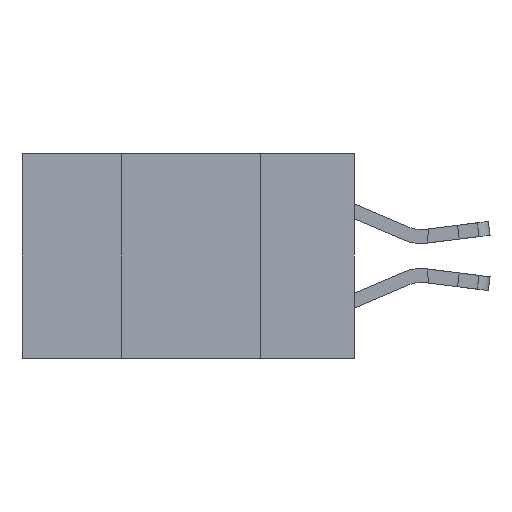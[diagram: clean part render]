
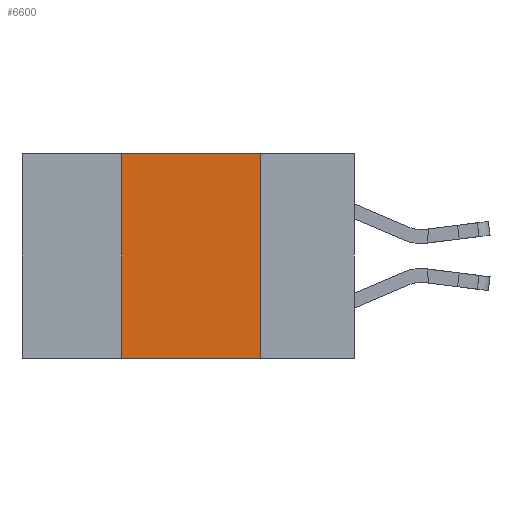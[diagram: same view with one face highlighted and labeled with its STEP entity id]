
A CAD part, left-side view. The second image highlights one B-rep face of the part: STEP entity #6600.
In plain terms, the highlighted planar face has unit normal (-1, 0, 0).
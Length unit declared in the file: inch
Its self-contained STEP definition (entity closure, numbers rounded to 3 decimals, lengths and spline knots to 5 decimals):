
#204 = CARTESIAN_POINT ( 'NONE',  ( 0., 0.6, 0. ) ) ;
#1066 = PLANE ( 'NONE',  #12484 ) ;
#1134 = CARTESIAN_POINT ( 'NONE',  ( 0., 0.42, -0.37 ) ) ;
#1773 = ORIENTED_EDGE ( 'NONE', *, *, #10359, .F. ) ;
#2123 = CARTESIAN_POINT ( 'NONE',  ( 0., 0.6, 0. ) ) ;
#2217 = VERTEX_POINT ( 'NONE', #1134 ) ;
#2220 = LINE ( 'NONE', #12725, #7137 ) ;
#2248 = EDGE_CURVE ( 'NONE', #2217, #8359, #2408, .T. ) ;
#2329 = EDGE_CURVE ( 'NONE', #2217, #6761, #12597, .T. ) ;
#2330 = DIRECTION ( 'NONE',  ( 0., -1., 0. ) ) ;
#2408 = LINE ( 'NONE', #5326, #4880 ) ;
#2549 = FACE_OUTER_BOUND ( 'NONE', #2796, .T. ) ;
#2796 = EDGE_LOOP ( 'NONE', ( #1773, #10125, #4559, #6039 ) ) ;
#3170 = DIRECTION ( 'NONE',  ( 0., 0., -1. ) ) ;
#4559 = ORIENTED_EDGE ( 'NONE', *, *, #2329, .F. ) ;
#4647 = LINE ( 'NONE', #204, #12364 ) ;
#4880 = VECTOR ( 'NONE', #7467, 39.37008 ) ;
#5326 = CARTESIAN_POINT ( 'NONE',  ( 0., 0.6, -0.37 ) ) ;
#5507 = CARTESIAN_POINT ( 'NONE',  ( 0., 0.42, -0.37 ) ) ;
#6039 = ORIENTED_EDGE ( 'NONE', *, *, #2248, .T. ) ;
#6412 = DIRECTION ( 'NONE',  ( 0., 0., -1. ) ) ;
#6554 = DIRECTION ( 'NONE',  ( 0., 0., 1. ) ) ;
#6600 = ADVANCED_FACE ( 'NONE', ( #2549 ), #1066, .F. ) ;
#6761 = VERTEX_POINT ( 'NONE', #11802 ) ;
#7137 = VECTOR ( 'NONE', #6412, 39.37008 ) ;
#7467 = DIRECTION ( 'NONE',  ( 0., -1., 0. ) ) ;
#8359 = VERTEX_POINT ( 'NONE', #10468 ) ;
#9397 = CARTESIAN_POINT ( 'NONE',  ( 0., 0.17, 0. ) ) ;
#9456 = DIRECTION ( 'NONE',  ( 1., 0., 0. ) ) ;
#9756 = EDGE_CURVE ( 'NONE', #6761, #10270, #4647, .T. ) ;
#10125 = ORIENTED_EDGE ( 'NONE', *, *, #9756, .F. ) ;
#10270 = VERTEX_POINT ( 'NONE', #9397 ) ;
#10359 = EDGE_CURVE ( 'NONE', #10270, #8359, #2220, .T. ) ;
#10468 = CARTESIAN_POINT ( 'NONE',  ( 0., 0.17, -0.37 ) ) ;
#11802 = CARTESIAN_POINT ( 'NONE',  ( 0., 0.42, 0. ) ) ;
#11922 = VECTOR ( 'NONE', #6554, 39.37008 ) ;
#12364 = VECTOR ( 'NONE', #2330, 39.37008 ) ;
#12484 = AXIS2_PLACEMENT_3D ( 'NONE', #2123, #9456, #3170 ) ;
#12597 = LINE ( 'NONE', #5507, #11922 ) ;
#12725 = CARTESIAN_POINT ( 'NONE',  ( 0., 0.17, -0.37 ) ) ;
